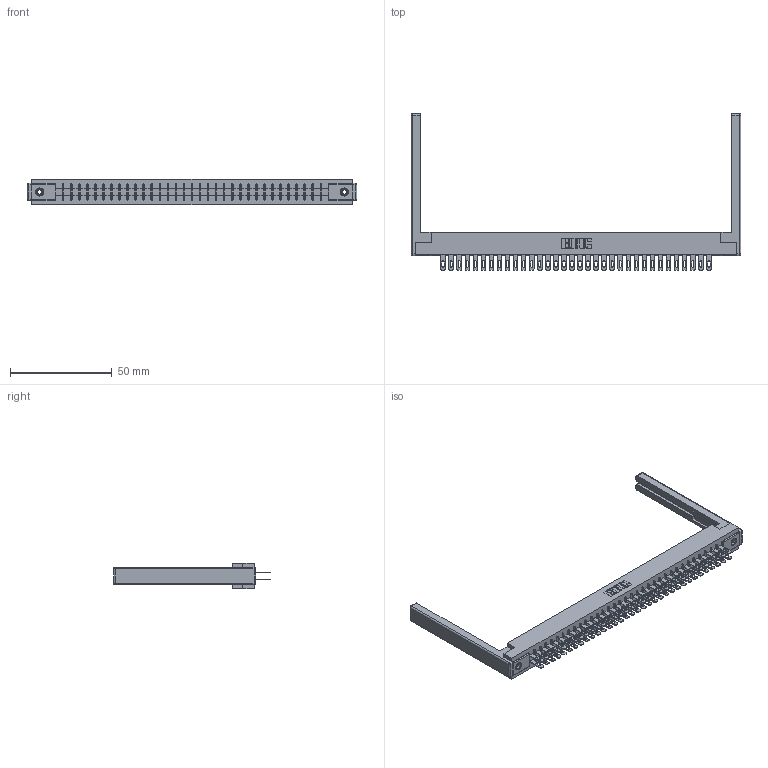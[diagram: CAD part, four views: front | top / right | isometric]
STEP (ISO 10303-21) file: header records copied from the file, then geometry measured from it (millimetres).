
FILE_DESCRIPTION (( 'STEP AP203' ), '1' );
FILE_NAME ('355-068-500-268.STEP', '2019-09-12T16:03:00', ( '' ), ( '' ), 'SwSTEP 2.0', 'SolidWorks 2016', '' );
FILE_SCHEMA (( 'CONFIG_CONTROL_DESIGN' ));
Length unit declared in the file: inch
Products named in the file (5): 355-068-500-268; 305-290-001_500; 305 Part_.156 Dia; 345-250-001_345-250-001-102; 307-220-068
Assembly tree (73 placements, depth 2):
  355-068-500-268
    305 Part_.156 Dia
    305-290-001_500  x68
    345-250-001_345-250-001-102  x2
    307-220-068  x2
Bounding box: 162.15 x 77.14 x 12.7 mm (x, y, z)
Volume: 21462.9 mm3; surface area: 26849.9 mm2
Topology: 73 solids, 73 shells, 3670 faces, 10464 edges, 6772 vertices
Faces by surface type: plane 2060, cylinder 1450, sphere 144, cone 12, torus 4
Entity records: 40568 total; most frequent: CARTESIAN_POINT 6685, ORIENTED_EDGE 6626, DIRECTION 6495, EDGE_CURVE 3313, VECTOR 2659, LINE 2659, VERTEX_POINT 2108, AXIS2_PLACEMENT_3D 1918
